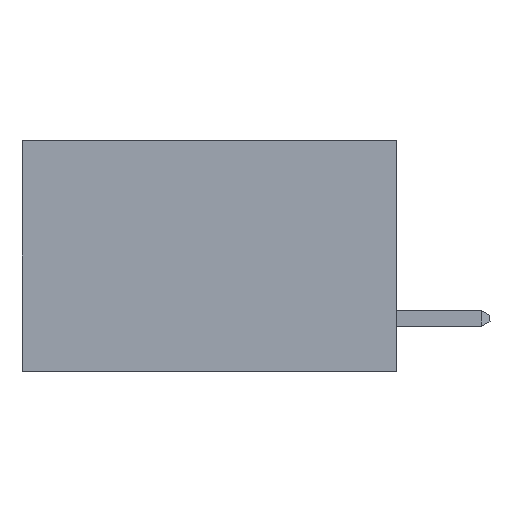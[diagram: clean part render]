
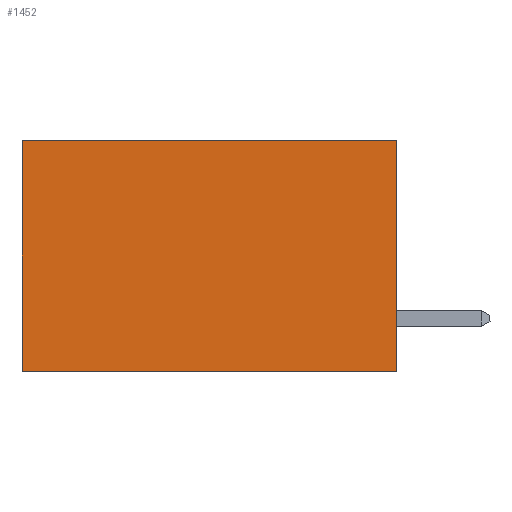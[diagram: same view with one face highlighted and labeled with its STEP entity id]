
A CAD part, left-side view. The second image highlights one B-rep face of the part: STEP entity #1452.
In plain terms, the highlighted planar face has unit normal (-1, 0, 0).
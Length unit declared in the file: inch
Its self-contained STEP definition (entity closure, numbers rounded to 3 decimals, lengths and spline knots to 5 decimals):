
#158 = DIRECTION ( 'NONE',  ( 0., 0., -1. ) ) ;
#194 = DIRECTION ( 'NONE',  ( 1., 0., 0. ) ) ;
#944 = DIRECTION ( 'NONE',  ( 0., 1., 0. ) ) ;
#1158 = EDGE_CURVE ( 'NONE', #5051, #2469, #8425, .T. ) ;
#1285 = VERTEX_POINT ( 'NONE', #2318 ) ;
#1452 = ADVANCED_FACE ( 'NONE', ( #2605 ), #5599, .F. ) ;
#1652 = CARTESIAN_POINT ( 'NONE',  ( 0.298, 0., 0. ) ) ;
#1878 = ORIENTED_EDGE ( 'NONE', *, *, #4301, .F. ) ;
#1900 = VECTOR ( 'NONE', #944, 39.37008 ) ;
#2318 = CARTESIAN_POINT ( 'NONE',  ( 0.298, 0., 0. ) ) ;
#2450 = ORIENTED_EDGE ( 'NONE', *, *, #1158, .T. ) ;
#2469 = VERTEX_POINT ( 'NONE', #6839 ) ;
#2605 = FACE_OUTER_BOUND ( 'NONE', #3982, .T. ) ;
#2845 = ORIENTED_EDGE ( 'NONE', *, *, #3482, .F. ) ;
#3197 = DIRECTION ( 'NONE',  ( 0., 1., 0. ) ) ;
#3482 = EDGE_CURVE ( 'NONE', #7250, #2469, #4158, .T. ) ;
#3545 = VECTOR ( 'NONE', #7921, 39.37008 ) ;
#3982 = EDGE_LOOP ( 'NONE', ( #2450, #2845, #1878, #10684 ) ) ;
#4048 = CARTESIAN_POINT ( 'NONE',  ( 0.298, 0., 0. ) ) ;
#4158 = LINE ( 'NONE', #5465, #1900 ) ;
#4301 = EDGE_CURVE ( 'NONE', #1285, #7250, #4775, .T. ) ;
#4775 = LINE ( 'NONE', #6710, #8834 ) ;
#4920 = CARTESIAN_POINT ( 'NONE',  ( 0.298, 0.6, 0. ) ) ;
#4947 = CARTESIAN_POINT ( 'NONE',  ( 0.298, 0., -0.37 ) ) ;
#5051 = VERTEX_POINT ( 'NONE', #5350 ) ;
#5350 = CARTESIAN_POINT ( 'NONE',  ( 0.298, 0.6, 0. ) ) ;
#5465 = CARTESIAN_POINT ( 'NONE',  ( 0.298, 0., -0.37 ) ) ;
#5599 = PLANE ( 'NONE',  #5639 ) ;
#5639 = AXIS2_PLACEMENT_3D ( 'NONE', #1652, #194, #158 ) ;
#6710 = CARTESIAN_POINT ( 'NONE',  ( 0.298, 0., 0. ) ) ;
#6839 = CARTESIAN_POINT ( 'NONE',  ( 0.298, 0.6, -0.37 ) ) ;
#7249 = VECTOR ( 'NONE', #3197, 39.37008 ) ;
#7250 = VERTEX_POINT ( 'NONE', #4947 ) ;
#7921 = DIRECTION ( 'NONE',  ( 0., 0., -1. ) ) ;
#8425 = LINE ( 'NONE', #4920, #3545 ) ;
#8834 = VECTOR ( 'NONE', #10228, 39.37008 ) ;
#9034 = EDGE_CURVE ( 'NONE', #1285, #5051, #10223, .T. ) ;
#10223 = LINE ( 'NONE', #4048, #7249 ) ;
#10228 = DIRECTION ( 'NONE',  ( 0., 0., -1. ) ) ;
#10684 = ORIENTED_EDGE ( 'NONE', *, *, #9034, .T. ) ;
